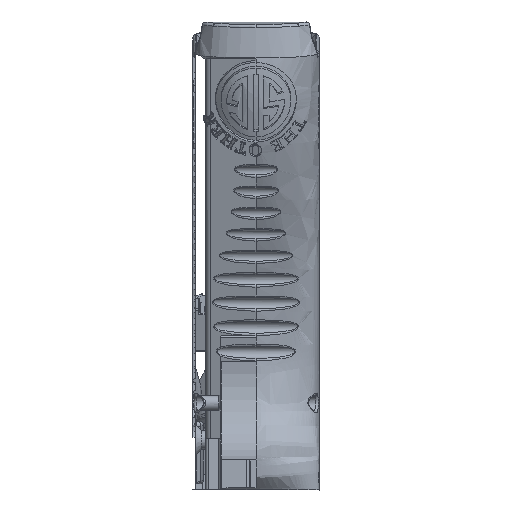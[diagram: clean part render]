
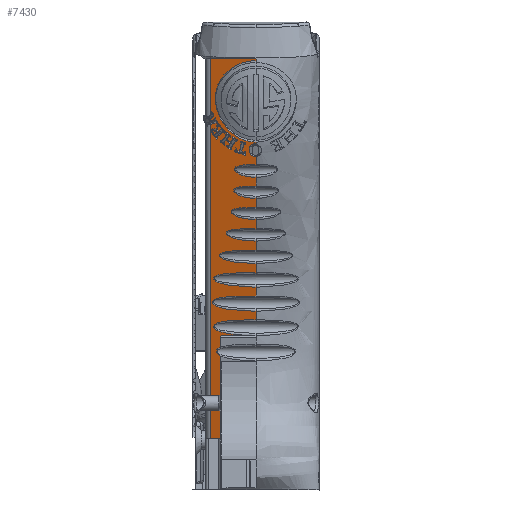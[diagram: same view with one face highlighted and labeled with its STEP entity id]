
A CAD part, left-side view. The second image highlights one B-rep face of the part: STEP entity #7430.
In plain terms, the highlighted planar face has unit normal (0.951, 0, 0.309).
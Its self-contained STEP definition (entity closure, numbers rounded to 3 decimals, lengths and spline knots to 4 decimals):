
#3263 = CARTESIAN_POINT ( 'NONE',  ( 2.0746, 0.37, -3.8765 ) ) ;
#3782 = VERTEX_POINT ( 'NONE', #53636 ) ;
#7430 = ADVANCED_FACE ( 'NONE', ( #33173 ), #63477, .F. ) ;
#8948 = CARTESIAN_POINT ( 'NONE',  ( 0.9499, 0.37, -0.4151 ) ) ;
#22015 = EDGE_CURVE ( 'NONE', #103089, #88847, #78208, .T. ) ;
#23102 = DIRECTION ( 'NONE',  ( -0.951, 0., -0.309 ) ) ;
#29042 = ORIENTED_EDGE ( 'NONE', *, *, #76822, .F. ) ;
#29670 = CARTESIAN_POINT ( 'NONE',  ( 1.9466, 0., -3.4826 ) ) ;
#32982 = DIRECTION ( 'NONE',  ( 0.309, 0., -0.951 ) ) ;
#33173 = FACE_OUTER_BOUND ( 'NONE', #44687, .T. ) ;
#36014 = VERTEX_POINT ( 'NONE', #124061 ) ;
#37229 = AXIS2_PLACEMENT_3D ( 'NONE', #89647, #23102, #116418 ) ;
#41073 = LINE ( 'NONE', #3263, #145175 ) ;
#42422 = VECTOR ( 'NONE', #112115, 39.3701 ) ;
#44687 = EDGE_LOOP ( 'NONE', ( #157386, #120623, #165654, #103650, #29042, #148209 ) ) ;
#53636 = CARTESIAN_POINT ( 'NONE',  ( 1.9466, 0.37, -3.4826 ) ) ;
#58794 = VERTEX_POINT ( 'NONE', #8948 ) ;
#59264 = LINE ( 'NONE', #132730, #176112 ) ;
#63477 = PLANE ( 'NONE',  #37229 ) ;
#76822 = EDGE_CURVE ( 'NONE', #36014, #103089, #59264, .T. ) ;
#77919 = DIRECTION ( 'NONE',  ( 0.309, 0., -0.951 ) ) ;
#78208 = LINE ( 'NONE', #140315, #139959 ) ;
#79163 = VECTOR ( 'NONE', #77919, 39.3701 ) ;
#84848 = LINE ( 'NONE', #152481, #42422 ) ;
#86734 = EDGE_CURVE ( 'NONE', #88847, #58794, #84848, .T. ) ;
#88847 = VERTEX_POINT ( 'NONE', #120420 ) ;
#89647 = CARTESIAN_POINT ( 'NONE',  ( 2.0746, 0., -3.8765 ) ) ;
#99697 = EDGE_CURVE ( 'NONE', #58794, #3782, #41073, .T. ) ;
#100094 = VERTEX_POINT ( 'NONE', #103569 ) ;
#103089 = VERTEX_POINT ( 'NONE', #120148 ) ;
#103569 = CARTESIAN_POINT ( 'NONE',  ( 1.9466, 0.0001, -3.4826 ) ) ;
#103650 = ORIENTED_EDGE ( 'NONE', *, *, #22015, .F. ) ;
#112115 = DIRECTION ( 'NONE',  ( 0., 1., 0. ) ) ;
#116418 = DIRECTION ( 'NONE',  ( -0.309, 0., 0.951 ) ) ;
#120148 = CARTESIAN_POINT ( 'NONE',  ( 2.0809, -0.37, -3.896 ) ) ;
#120420 = CARTESIAN_POINT ( 'NONE',  ( 0.9499, -0.37, -0.4151 ) ) ;
#120623 = ORIENTED_EDGE ( 'NONE', *, *, #99697, .F. ) ;
#121235 = CARTESIAN_POINT ( 'NONE',  ( 2.0746, 0.0001, -3.8765 ) ) ;
#124061 = CARTESIAN_POINT ( 'NONE',  ( 2.0809, 0.0001, -3.896 ) ) ;
#132526 = LINE ( 'NONE', #121235, #79163 ) ;
#132730 = CARTESIAN_POINT ( 'NONE',  ( 2.0809, 0., -3.896 ) ) ;
#137759 = DIRECTION ( 'NONE',  ( 0., -1., 0. ) ) ;
#139959 = VECTOR ( 'NONE', #166430, 39.3701 ) ;
#140315 = CARTESIAN_POINT ( 'NONE',  ( 2.0746, -0.37, -3.8765 ) ) ;
#145175 = VECTOR ( 'NONE', #32982, 39.3701 ) ;
#145214 = DIRECTION ( 'NONE',  ( 0., -1., 0. ) ) ;
#145560 = EDGE_CURVE ( 'NONE', #3782, #100094, #166784, .T. ) ;
#148209 = ORIENTED_EDGE ( 'NONE', *, *, #149067, .F. ) ;
#149067 = EDGE_CURVE ( 'NONE', #100094, #36014, #132526, .T. ) ;
#152481 = CARTESIAN_POINT ( 'NONE',  ( 0.9499, 0., -0.4151 ) ) ;
#157386 = ORIENTED_EDGE ( 'NONE', *, *, #145560, .F. ) ;
#158285 = VECTOR ( 'NONE', #137759, 39.3701 ) ;
#165654 = ORIENTED_EDGE ( 'NONE', *, *, #86734, .F. ) ;
#166430 = DIRECTION ( 'NONE',  ( -0.309, 0., 0.951 ) ) ;
#166784 = LINE ( 'NONE', #29670, #158285 ) ;
#176112 = VECTOR ( 'NONE', #145214, 39.3701 ) ;
